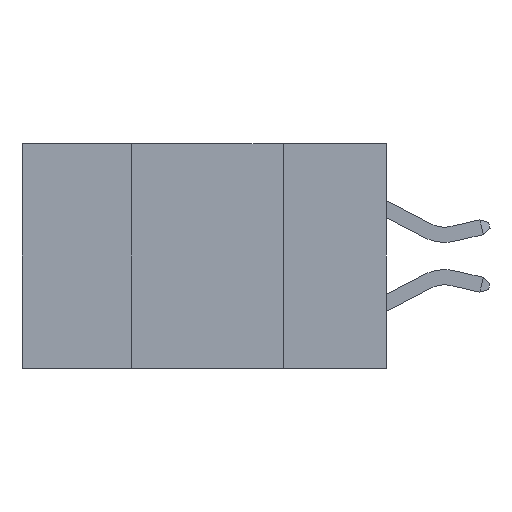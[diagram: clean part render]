
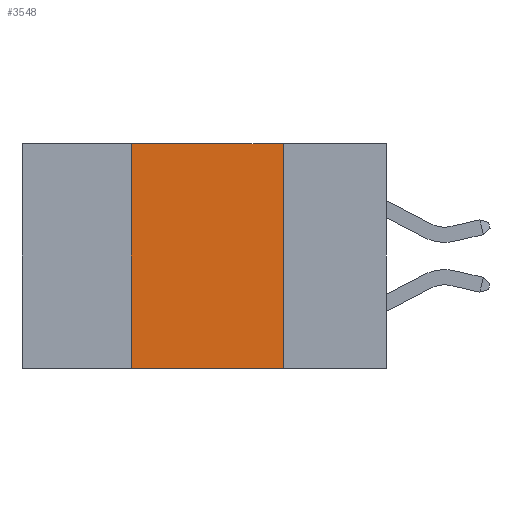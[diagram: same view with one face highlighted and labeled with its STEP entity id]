
A CAD part, left-side view. The second image highlights one B-rep face of the part: STEP entity #3548.
In plain terms, the highlighted planar face has unit normal (-1, 0, 0).
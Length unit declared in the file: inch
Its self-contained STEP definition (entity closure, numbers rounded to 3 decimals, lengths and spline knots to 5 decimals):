
#42 = EDGE_CURVE ( 'NONE', #7347, #5016, #8418, .T. ) ;
#284 = ORIENTED_EDGE ( 'NONE', *, *, #6912, .F. ) ;
#651 = LINE ( 'NONE', #6337, #6139 ) ;
#786 = EDGE_CURVE ( 'NONE', #6456, #12363, #651, .T. ) ;
#794 = DIRECTION ( 'NONE',  ( 0., 0., 1. ) ) ;
#1479 = LINE ( 'NONE', #3477, #6618 ) ;
#2733 = ORIENTED_EDGE ( 'NONE', *, *, #11724, .F. ) ;
#2855 = EDGE_LOOP ( 'NONE', ( #284, #3056, #2733, #10666 ) ) ;
#3056 = ORIENTED_EDGE ( 'NONE', *, *, #786, .F. ) ;
#3189 = CARTESIAN_POINT ( 'NONE',  ( 0., 0.17, -0.37 ) ) ;
#3388 = VECTOR ( 'NONE', #12315, 39.37008 ) ;
#3477 = CARTESIAN_POINT ( 'NONE',  ( 0., 0.17, 0. ) ) ;
#3548 = ADVANCED_FACE ( 'NONE', ( #3842 ), #12385, .F. ) ;
#3692 = CARTESIAN_POINT ( 'NONE',  ( 0., 0.42, -0.37 ) ) ;
#3842 = FACE_OUTER_BOUND ( 'NONE', #2855, .T. ) ;
#3945 = VECTOR ( 'NONE', #794, 39.37008 ) ;
#4476 = CARTESIAN_POINT ( 'NONE',  ( 0., 0.6, -0.37 ) ) ;
#4610 = CARTESIAN_POINT ( 'NONE',  ( 0., 0.17, 0. ) ) ;
#5016 = VERTEX_POINT ( 'NONE', #3189 ) ;
#5147 = DIRECTION ( 'NONE',  ( 0., 0., -1. ) ) ;
#5526 = DIRECTION ( 'NONE',  ( 1., 0., 0. ) ) ;
#6139 = VECTOR ( 'NONE', #6381, 39.37008 ) ;
#6337 = CARTESIAN_POINT ( 'NONE',  ( 0., 0.6, 0. ) ) ;
#6381 = DIRECTION ( 'NONE',  ( 0., -1., 0. ) ) ;
#6456 = VERTEX_POINT ( 'NONE', #8327 ) ;
#6618 = VECTOR ( 'NONE', #7619, 39.37008 ) ;
#6648 = LINE ( 'NONE', #12679, #3945 ) ;
#6816 = AXIS2_PLACEMENT_3D ( 'NONE', #12278, #5526, #5147 ) ;
#6912 = EDGE_CURVE ( 'NONE', #12363, #5016, #1479, .T. ) ;
#7347 = VERTEX_POINT ( 'NONE', #3692 ) ;
#7619 = DIRECTION ( 'NONE',  ( 0., 0., -1. ) ) ;
#8327 = CARTESIAN_POINT ( 'NONE',  ( 0., 0.42, 0. ) ) ;
#8418 = LINE ( 'NONE', #4476, #3388 ) ;
#10666 = ORIENTED_EDGE ( 'NONE', *, *, #42, .T. ) ;
#11724 = EDGE_CURVE ( 'NONE', #7347, #6456, #6648, .T. ) ;
#12278 = CARTESIAN_POINT ( 'NONE',  ( 0., 0.6, 0. ) ) ;
#12315 = DIRECTION ( 'NONE',  ( 0., -1., 0. ) ) ;
#12363 = VERTEX_POINT ( 'NONE', #4610 ) ;
#12385 = PLANE ( 'NONE',  #6816 ) ;
#12679 = CARTESIAN_POINT ( 'NONE',  ( 0., 0.42, 0. ) ) ;
